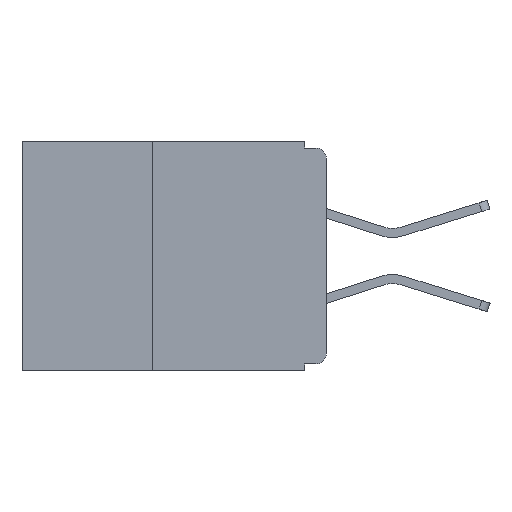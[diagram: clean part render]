
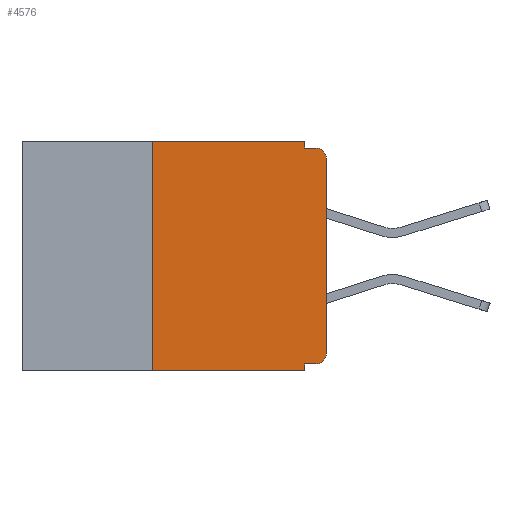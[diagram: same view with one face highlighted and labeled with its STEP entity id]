
A CAD part, left-side view. The second image highlights one B-rep face of the part: STEP entity #4576.
In plain terms, the highlighted planar face has unit normal (-1, 0, 0).
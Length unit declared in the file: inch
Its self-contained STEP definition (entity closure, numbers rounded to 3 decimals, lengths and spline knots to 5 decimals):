
#456 = VERTEX_POINT ( 'NONE', #7805 ) ;
#763 = AXIS2_PLACEMENT_3D ( 'NONE', #8998, #8404, #11319 ) ;
#1150 = DIRECTION ( 'NONE',  ( 0., 0., 1. ) ) ;
#1413 = EDGE_CURVE ( 'NONE', #8411, #456, #9327, .T. ) ;
#1449 = CARTESIAN_POINT ( 'NONE',  ( 0., 0.031, -0.33 ) ) ;
#1563 = VECTOR ( 'NONE', #8558, 39.37008 ) ;
#1636 = EDGE_CURVE ( 'NONE', #10955, #5496, #5851, .T. ) ;
#1810 = FACE_OUTER_BOUND ( 'NONE', #4216, .T. ) ;
#1910 = LINE ( 'NONE', #8811, #1563 ) ;
#1992 = VECTOR ( 'NONE', #4535, 39.37008 ) ;
#2059 = VECTOR ( 'NONE', #10988, 39.37008 ) ;
#2066 = VERTEX_POINT ( 'NONE', #12060 ) ;
#2186 = LINE ( 'NONE', #8606, #1992 ) ;
#2231 = VECTOR ( 'NONE', #7928, 39.37008 ) ;
#2269 = LINE ( 'NONE', #11415, #2059 ) ;
#2367 = ORIENTED_EDGE ( 'NONE', *, *, #6245, .F. ) ;
#2495 = LINE ( 'NONE', #8016, #2231 ) ;
#2637 = VECTOR ( 'NONE', #1150, 39.37008 ) ;
#2937 = ORIENTED_EDGE ( 'NONE', *, *, #1413, .T. ) ;
#2951 = VERTEX_POINT ( 'NONE', #10670 ) ;
#2959 = EDGE_CURVE ( 'NONE', #3124, #5496, #9971, .T. ) ;
#3037 = LINE ( 'NONE', #11592, #2637 ) ;
#3079 = VERTEX_POINT ( 'NONE', #11962 ) ;
#3124 = VERTEX_POINT ( 'NONE', #11080 ) ;
#3459 = ORIENTED_EDGE ( 'NONE', *, *, #7571, .T. ) ;
#3703 = AXIS2_PLACEMENT_3D ( 'NONE', #6822, #5984, #7052 ) ;
#3775 = CARTESIAN_POINT ( 'NONE',  ( 0., 0.25, 0. ) ) ;
#4012 = EDGE_CURVE ( 'NONE', #3124, #5239, #3037, .T. ) ;
#4036 = DIRECTION ( 'NONE',  ( 0., -1., 0. ) ) ;
#4126 = ORIENTED_EDGE ( 'NONE', *, *, #8916, .T. ) ;
#4216 = EDGE_LOOP ( 'NONE', ( #4126, #3459, #7201, #6279, #7715, #8906, #10062, #10256, #2367, #2937 ) ) ;
#4413 = CARTESIAN_POINT ( 'NONE',  ( 0., 0.031, 0. ) ) ;
#4500 = EDGE_CURVE ( 'NONE', #8509, #3079, #2495, .T. ) ;
#4535 = DIRECTION ( 'NONE',  ( 0., -1., 0. ) ) ;
#4576 = ADVANCED_FACE ( 'NONE', ( #1810 ), #7149, .F. ) ;
#4814 = CARTESIAN_POINT ( 'NONE',  ( 0., 0.437, -0.33 ) ) ;
#5239 = VERTEX_POINT ( 'NONE', #3775 ) ;
#5496 = VERTEX_POINT ( 'NONE', #1449 ) ;
#5526 = VECTOR ( 'NONE', #8504, 39.37008 ) ;
#5651 = VECTOR ( 'NONE', #10215, 39.37008 ) ;
#5799 = LINE ( 'NONE', #10428, #5651 ) ;
#5851 = LINE ( 'NONE', #6515, #5526 ) ;
#5984 = DIRECTION ( 'NONE',  ( 1., 0., 0. ) ) ;
#6245 = EDGE_CURVE ( 'NONE', #8411, #10955, #5799, .T. ) ;
#6279 = ORIENTED_EDGE ( 'NONE', *, *, #4500, .F. ) ;
#6515 = CARTESIAN_POINT ( 'NONE',  ( 0., 0.031, -0.33 ) ) ;
#6822 = CARTESIAN_POINT ( 'NONE',  ( 0., 0.437, 0. ) ) ;
#7052 = DIRECTION ( 'NONE',  ( 0., 0., -1. ) ) ;
#7149 = PLANE ( 'NONE',  #3703 ) ;
#7201 = ORIENTED_EDGE ( 'NONE', *, *, #9896, .F. ) ;
#7419 = CARTESIAN_POINT ( 'NONE',  ( 0., 0.031, -0.32 ) ) ;
#7571 = EDGE_CURVE ( 'NONE', #2951, #2066, #11749, .T. ) ;
#7715 = ORIENTED_EDGE ( 'NONE', *, *, #8223, .F. ) ;
#7805 = CARTESIAN_POINT ( 'NONE',  ( 0., 0., -0.305 ) ) ;
#7928 = DIRECTION ( 'NONE',  ( 0., 0., -1. ) ) ;
#8016 = CARTESIAN_POINT ( 'NONE',  ( 0., 0.031, 0. ) ) ;
#8223 = EDGE_CURVE ( 'NONE', #5239, #8509, #2186, .T. ) ;
#8404 = DIRECTION ( 'NONE',  ( -1., 0., 0. ) ) ;
#8411 = VERTEX_POINT ( 'NONE', #8773 ) ;
#8504 = DIRECTION ( 'NONE',  ( 0., 0., -1. ) ) ;
#8509 = VERTEX_POINT ( 'NONE', #4413 ) ;
#8558 = DIRECTION ( 'NONE',  ( 0., -1., 0. ) ) ;
#8606 = CARTESIAN_POINT ( 'NONE',  ( 0., 0.437, 0. ) ) ;
#8749 = DIRECTION ( 'NONE',  ( 0., 0., -1. ) ) ;
#8773 = CARTESIAN_POINT ( 'NONE',  ( 0., 0.015, -0.32 ) ) ;
#8811 = CARTESIAN_POINT ( 'NONE',  ( 0., 0., -0.01 ) ) ;
#8897 = DIRECTION ( 'NONE',  ( -1., 0., 0. ) ) ;
#8900 = CARTESIAN_POINT ( 'NONE',  ( 0., 0.015, -0.025 ) ) ;
#8906 = ORIENTED_EDGE ( 'NONE', *, *, #4012, .F. ) ;
#8916 = EDGE_CURVE ( 'NONE', #456, #2951, #2269, .T. ) ;
#8998 = CARTESIAN_POINT ( 'NONE',  ( 0., 0.015, -0.305 ) ) ;
#9327 = CIRCLE ( 'NONE', #763, 0.015 ) ;
#9896 = EDGE_CURVE ( 'NONE', #3079, #2066, #1910, .T. ) ;
#9921 = VECTOR ( 'NONE', #4036, 39.37008 ) ;
#9971 = LINE ( 'NONE', #4814, #9921 ) ;
#10062 = ORIENTED_EDGE ( 'NONE', *, *, #2959, .T. ) ;
#10147 = AXIS2_PLACEMENT_3D ( 'NONE', #8900, #8897, #8749 ) ;
#10215 = DIRECTION ( 'NONE',  ( 0., 1., 0. ) ) ;
#10256 = ORIENTED_EDGE ( 'NONE', *, *, #1636, .F. ) ;
#10428 = CARTESIAN_POINT ( 'NONE',  ( 0., 0., -0.32 ) ) ;
#10670 = CARTESIAN_POINT ( 'NONE',  ( 0., 0., -0.025 ) ) ;
#10955 = VERTEX_POINT ( 'NONE', #7419 ) ;
#10988 = DIRECTION ( 'NONE',  ( 0., 0., 1. ) ) ;
#11080 = CARTESIAN_POINT ( 'NONE',  ( 0., 0.25, -0.33 ) ) ;
#11319 = DIRECTION ( 'NONE',  ( 0., 0., -1. ) ) ;
#11415 = CARTESIAN_POINT ( 'NONE',  ( 0., 0., 0. ) ) ;
#11592 = CARTESIAN_POINT ( 'NONE',  ( 0., 0.25, -0.33 ) ) ;
#11749 = CIRCLE ( 'NONE', #10147, 0.015 ) ;
#11962 = CARTESIAN_POINT ( 'NONE',  ( 0., 0.031, -0.01 ) ) ;
#12060 = CARTESIAN_POINT ( 'NONE',  ( 0., 0.015, -0.01 ) ) ;
